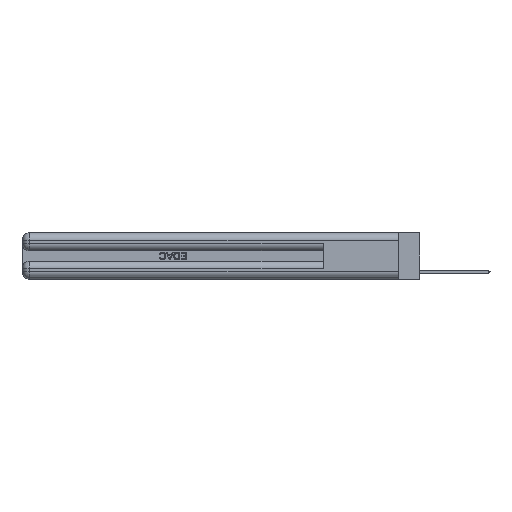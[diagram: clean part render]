
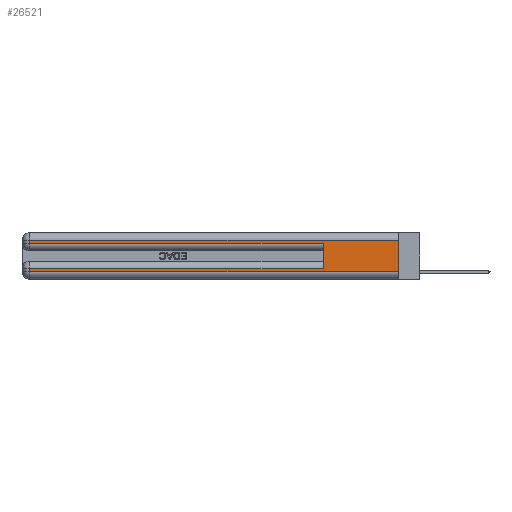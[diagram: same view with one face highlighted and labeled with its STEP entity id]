
A CAD part, left-side view. The second image highlights one B-rep face of the part: STEP entity #26521.
In plain terms, the highlighted planar face has unit normal (-1, 0, 0).
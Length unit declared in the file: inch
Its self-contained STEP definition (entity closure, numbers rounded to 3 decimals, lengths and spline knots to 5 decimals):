
#576 = EDGE_CURVE ( 'NONE', #6137, #25605, #26646, .T. ) ;
#1856 = CARTESIAN_POINT ( 'NONE',  ( 0., 2.94, 0.285 ) ) ;
#2082 = EDGE_CURVE ( 'NONE', #25605, #31215, #24742, .T. ) ;
#2425 = ORIENTED_EDGE ( 'NONE', *, *, #28719, .T. ) ;
#3071 = EDGE_CURVE ( 'NONE', #31215, #11626, #28055, .T. ) ;
#3108 = ORIENTED_EDGE ( 'NONE', *, *, #13108, .T. ) ;
#3245 = VECTOR ( 'NONE', #24321, 39.37008 ) ;
#3481 = CARTESIAN_POINT ( 'NONE',  ( 0., 2.94, 0.37 ) ) ;
#4391 = LINE ( 'NONE', #24739, #3245 ) ;
#5085 = VERTEX_POINT ( 'NONE', #24544 ) ;
#6114 = AXIS2_PLACEMENT_3D ( 'NONE', #24204, #26594, #19330 ) ;
#6137 = VERTEX_POINT ( 'NONE', #24764 ) ;
#6592 = CARTESIAN_POINT ( 'NONE',  ( 0., 0., 0.37 ) ) ;
#7790 = CARTESIAN_POINT ( 'NONE',  ( 0., 0., 0.285 ) ) ;
#7959 = ORIENTED_EDGE ( 'NONE', *, *, #29988, .T. ) ;
#8627 = VECTOR ( 'NONE', #11014, 39.37008 ) ;
#8659 = LINE ( 'NONE', #25051, #12840 ) ;
#9264 = EDGE_CURVE ( 'NONE', #30022, #11626, #11503, .T. ) ;
#10291 = CARTESIAN_POINT ( 'NONE',  ( 0., 2.94, 0.37 ) ) ;
#11014 = DIRECTION ( 'NONE',  ( 0., 0., -1. ) ) ;
#11503 = LINE ( 'NONE', #21489, #13451 ) ;
#11626 = VERTEX_POINT ( 'NONE', #14307 ) ;
#11947 = CARTESIAN_POINT ( 'NONE',  ( 0., 0., 0.31 ) ) ;
#12840 = VECTOR ( 'NONE', #15728, 39.37008 ) ;
#13108 = EDGE_CURVE ( 'NONE', #27373, #23107, #8659, .T. ) ;
#13451 = VECTOR ( 'NONE', #14352, 39.37008 ) ;
#13731 = DIRECTION ( 'NONE',  ( 0., 0., -1. ) ) ;
#14307 = CARTESIAN_POINT ( 'NONE',  ( 0., 0.6, 0.285 ) ) ;
#14352 = DIRECTION ( 'NONE',  ( 0., 0., 1. ) ) ;
#14662 = LINE ( 'NONE', #3481, #8627 ) ;
#14817 = ORIENTED_EDGE ( 'NONE', *, *, #3071, .T. ) ;
#15664 = VECTOR ( 'NONE', #19283, 39.37008 ) ;
#15728 = DIRECTION ( 'NONE',  ( 0., -1., 0. ) ) ;
#17345 = LINE ( 'NONE', #6592, #26056 ) ;
#17420 = CARTESIAN_POINT ( 'NONE',  ( 0., 0.6, 0.085 ) ) ;
#19283 = DIRECTION ( 'NONE',  ( 0., 1., 0. ) ) ;
#19330 = DIRECTION ( 'NONE',  ( 0., 0., -1. ) ) ;
#19457 = VECTOR ( 'NONE', #25119, 39.37008 ) ;
#20522 = VECTOR ( 'NONE', #29650, 39.37008 ) ;
#20596 = ORIENTED_EDGE ( 'NONE', *, *, #29780, .F. ) ;
#21097 = FACE_OUTER_BOUND ( 'NONE', #27332, .T. ) ;
#21489 = CARTESIAN_POINT ( 'NONE',  ( 0., 0.6, 0.145 ) ) ;
#21881 = ORIENTED_EDGE ( 'NONE', *, *, #9264, .F. ) ;
#23107 = VERTEX_POINT ( 'NONE', #31269 ) ;
#24204 = CARTESIAN_POINT ( 'NONE',  ( 0., 0., 0.37 ) ) ;
#24321 = DIRECTION ( 'NONE',  ( 0., 1., 0. ) ) ;
#24544 = CARTESIAN_POINT ( 'NONE',  ( 0., 2.94, 0.085 ) ) ;
#24739 = CARTESIAN_POINT ( 'NONE',  ( 0., 0., 0.085 ) ) ;
#24742 = LINE ( 'NONE', #10291, #19457 ) ;
#24764 = CARTESIAN_POINT ( 'NONE',  ( 0., 0., 0.31 ) ) ;
#25051 = CARTESIAN_POINT ( 'NONE',  ( 0., 0., 0.06 ) ) ;
#25119 = DIRECTION ( 'NONE',  ( 0., 0., -1. ) ) ;
#25205 = CARTESIAN_POINT ( 'NONE',  ( 0., 2.94, 0.31 ) ) ;
#25605 = VERTEX_POINT ( 'NONE', #25205 ) ;
#26056 = VECTOR ( 'NONE', #13731, 39.37008 ) ;
#26521 = ADVANCED_FACE ( 'NONE', ( #21097 ), #28708, .F. ) ;
#26594 = DIRECTION ( 'NONE',  ( 1., 0., 0. ) ) ;
#26646 = LINE ( 'NONE', #11947, #15664 ) ;
#27165 = ORIENTED_EDGE ( 'NONE', *, *, #2082, .T. ) ;
#27332 = EDGE_LOOP ( 'NONE', ( #20596, #28162, #27165, #14817, #21881, #7959, #2425, #3108 ) ) ;
#27373 = VERTEX_POINT ( 'NONE', #27917 ) ;
#27917 = CARTESIAN_POINT ( 'NONE',  ( 0., 2.94, 0.06 ) ) ;
#28055 = LINE ( 'NONE', #7790, #20522 ) ;
#28162 = ORIENTED_EDGE ( 'NONE', *, *, #576, .T. ) ;
#28708 = PLANE ( 'NONE',  #6114 ) ;
#28719 = EDGE_CURVE ( 'NONE', #5085, #27373, #14662, .T. ) ;
#29650 = DIRECTION ( 'NONE',  ( 0., -1., 0. ) ) ;
#29780 = EDGE_CURVE ( 'NONE', #6137, #23107, #17345, .T. ) ;
#29988 = EDGE_CURVE ( 'NONE', #30022, #5085, #4391, .T. ) ;
#30022 = VERTEX_POINT ( 'NONE', #17420 ) ;
#31215 = VERTEX_POINT ( 'NONE', #1856 ) ;
#31269 = CARTESIAN_POINT ( 'NONE',  ( 0., 0., 0.06 ) ) ;
